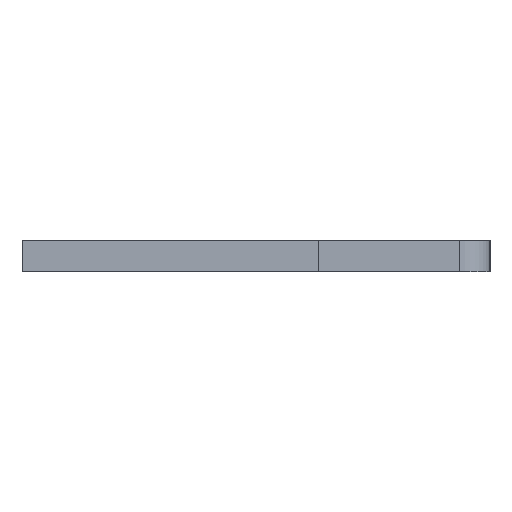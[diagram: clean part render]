
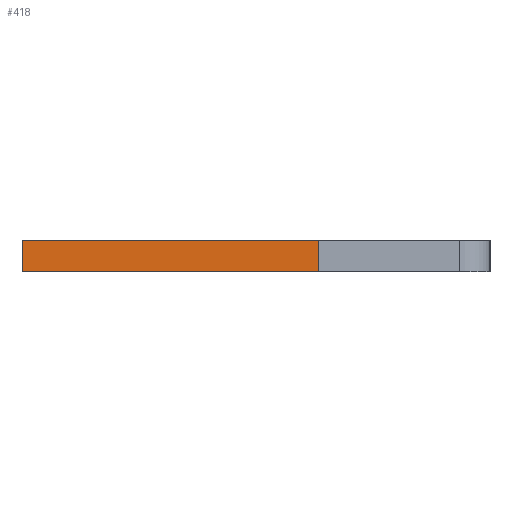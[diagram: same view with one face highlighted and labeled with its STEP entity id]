
A CAD part, left-side view. The second image highlights one B-rep face of the part: STEP entity #418.
In plain terms, the highlighted face is planar.
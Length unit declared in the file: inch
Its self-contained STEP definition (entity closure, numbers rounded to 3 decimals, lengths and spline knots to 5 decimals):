
#107 = VERTEX_POINT ( 'NONE', #1615 ) ;
#121 = EDGE_CURVE ( 'NONE', #1732, #107, #920, .T. ) ;
#139 = DIRECTION ( 'NONE',  ( 0., 1., 0. ) ) ;
#247 = ORIENTED_EDGE ( 'NONE', *, *, #121, .F. ) ;
#269 = AXIS2_PLACEMENT_3D ( 'NONE', #2306, #426, #1494 ) ;
#312 = CARTESIAN_POINT ( 'NONE',  ( 0.01, -0.04, -0.04 ) ) ;
#418 = ADVANCED_FACE ( 'NONE', ( #1640 ), #1483, .F. ) ;
#426 = DIRECTION ( 'NONE',  ( 0., 0., 1. ) ) ;
#532 = CARTESIAN_POINT ( 'NONE',  ( -0.01, 0.15, -0.04 ) ) ;
#564 = ORIENTED_EDGE ( 'NONE', *, *, #1761, .T. ) ;
#920 = LINE ( 'NONE', #2715, #1982 ) ;
#939 = EDGE_CURVE ( 'NONE', #1701, #2342, #1092, .T. ) ;
#1019 = VECTOR ( 'NONE', #1509, 39.37008 ) ;
#1027 = LINE ( 'NONE', #2470, #2087 ) ;
#1092 = LINE ( 'NONE', #1719, #1019 ) ;
#1339 = CARTESIAN_POINT ( 'NONE',  ( 0.01, 0.15, -0.04 ) ) ;
#1483 = PLANE ( 'NONE',  #269 ) ;
#1494 = DIRECTION ( 'NONE',  ( 1., 0., 0. ) ) ;
#1509 = DIRECTION ( 'NONE',  ( -1., 0., 0. ) ) ;
#1611 = VECTOR ( 'NONE', #2410, 39.37008 ) ;
#1615 = CARTESIAN_POINT ( 'NONE',  ( -0.01, 0.15, -0.04 ) ) ;
#1640 = FACE_OUTER_BOUND ( 'NONE', #2047, .T. ) ;
#1701 = VERTEX_POINT ( 'NONE', #312 ) ;
#1719 = CARTESIAN_POINT ( 'NONE',  ( 0.01, -0.04, -0.04 ) ) ;
#1732 = VERTEX_POINT ( 'NONE', #1339 ) ;
#1761 = EDGE_CURVE ( 'NONE', #2342, #107, #1936, .T. ) ;
#1833 = DIRECTION ( 'NONE',  ( -1., 0., 0. ) ) ;
#1936 = LINE ( 'NONE', #532, #1611 ) ;
#1982 = VECTOR ( 'NONE', #1833, 39.37008 ) ;
#2047 = EDGE_LOOP ( 'NONE', ( #564, #247, #2177, #2372 ) ) ;
#2087 = VECTOR ( 'NONE', #139, 39.37008 ) ;
#2177 = ORIENTED_EDGE ( 'NONE', *, *, #2581, .F. ) ;
#2306 = CARTESIAN_POINT ( 'NONE',  ( 0.01, 0.15, -0.04 ) ) ;
#2342 = VERTEX_POINT ( 'NONE', #2478 ) ;
#2372 = ORIENTED_EDGE ( 'NONE', *, *, #939, .T. ) ;
#2410 = DIRECTION ( 'NONE',  ( 0., 1., 0. ) ) ;
#2470 = CARTESIAN_POINT ( 'NONE',  ( 0.01, 0.15, -0.04 ) ) ;
#2478 = CARTESIAN_POINT ( 'NONE',  ( -0.01, -0.04, -0.04 ) ) ;
#2581 = EDGE_CURVE ( 'NONE', #1701, #1732, #1027, .T. ) ;
#2715 = CARTESIAN_POINT ( 'NONE',  ( 0.01, 0.15, -0.04 ) ) ;
